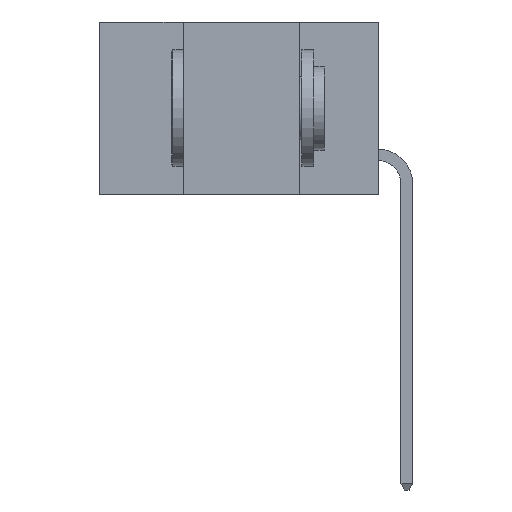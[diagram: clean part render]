
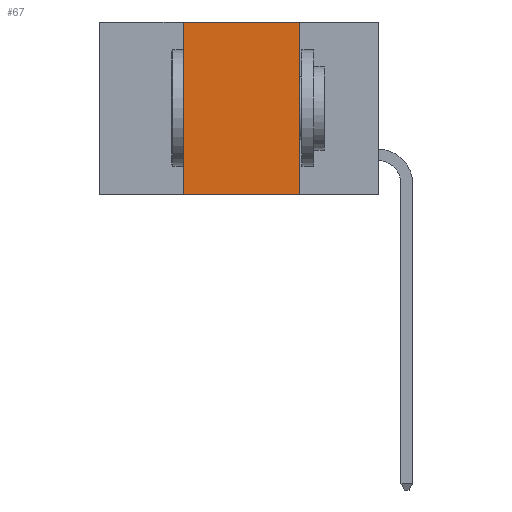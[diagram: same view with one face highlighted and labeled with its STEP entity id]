
A CAD part, left-side view. The second image highlights one B-rep face of the part: STEP entity #67.
In plain terms, the highlighted planar face has unit normal (-1, 0, 0).
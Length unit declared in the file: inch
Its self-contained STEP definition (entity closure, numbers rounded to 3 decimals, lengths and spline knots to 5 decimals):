
#67 = ADVANCED_FACE ( 'NONE', ( #15768 ), #16249, .F. ) ;
#291 = DIRECTION ( 'NONE',  ( 0., 0., -1. ) ) ;
#509 = LINE ( 'NONE', #733, #12382 ) ;
#733 = CARTESIAN_POINT ( 'NONE',  ( 0., 0.6, 0. ) ) ;
#1095 = ORIENTED_EDGE ( 'NONE', *, *, #23793, .F. ) ;
#4222 = DIRECTION ( 'NONE',  ( 1., 0., 0. ) ) ;
#6636 = CARTESIAN_POINT ( 'NONE',  ( 0., 0.6, -0.37 ) ) ;
#6650 = LINE ( 'NONE', #6636, #22644 ) ;
#7307 = EDGE_CURVE ( 'NONE', #18733, #16994, #9834, .T. ) ;
#7585 = DIRECTION ( 'NONE',  ( 0., 0., 1. ) ) ;
#7842 = LINE ( 'NONE', #12940, #23212 ) ;
#9834 = LINE ( 'NONE', #20109, #20930 ) ;
#9848 = EDGE_CURVE ( 'NONE', #16994, #19697, #509, .T. ) ;
#10142 = CARTESIAN_POINT ( 'NONE',  ( 0., 0.17, -0.37 ) ) ;
#10703 = ORIENTED_EDGE ( 'NONE', *, *, #19552, .T. ) ;
#12382 = VECTOR ( 'NONE', #15474, 39.37008 ) ;
#12640 = CARTESIAN_POINT ( 'NONE',  ( 0., 0.42, 0. ) ) ;
#12940 = CARTESIAN_POINT ( 'NONE',  ( 0., 0.17, -0.37 ) ) ;
#13645 = ORIENTED_EDGE ( 'NONE', *, *, #9848, .F. ) ;
#13785 = AXIS2_PLACEMENT_3D ( 'NONE', #26188, #4222, #24639 ) ;
#15474 = DIRECTION ( 'NONE',  ( 0., -1., 0. ) ) ;
#15527 = CARTESIAN_POINT ( 'NONE',  ( 0., 0.17, 0. ) ) ;
#15768 = FACE_OUTER_BOUND ( 'NONE', #24888, .T. ) ;
#16249 = PLANE ( 'NONE',  #13785 ) ;
#16994 = VERTEX_POINT ( 'NONE', #12640 ) ;
#18733 = VERTEX_POINT ( 'NONE', #24140 ) ;
#19168 = DIRECTION ( 'NONE',  ( 0., -1., 0. ) ) ;
#19318 = VERTEX_POINT ( 'NONE', #10142 ) ;
#19552 = EDGE_CURVE ( 'NONE', #18733, #19318, #6650, .T. ) ;
#19697 = VERTEX_POINT ( 'NONE', #15527 ) ;
#20109 = CARTESIAN_POINT ( 'NONE',  ( 0., 0.42, -0.37 ) ) ;
#20930 = VECTOR ( 'NONE', #7585, 39.37008 ) ;
#22644 = VECTOR ( 'NONE', #19168, 39.37008 ) ;
#23212 = VECTOR ( 'NONE', #291, 39.37008 ) ;
#23793 = EDGE_CURVE ( 'NONE', #19697, #19318, #7842, .T. ) ;
#24140 = CARTESIAN_POINT ( 'NONE',  ( 0., 0.42, -0.37 ) ) ;
#24639 = DIRECTION ( 'NONE',  ( 0., 0., -1. ) ) ;
#24888 = EDGE_LOOP ( 'NONE', ( #1095, #13645, #25325, #10703 ) ) ;
#25325 = ORIENTED_EDGE ( 'NONE', *, *, #7307, .F. ) ;
#26188 = CARTESIAN_POINT ( 'NONE',  ( 0., 0.6, 0. ) ) ;
